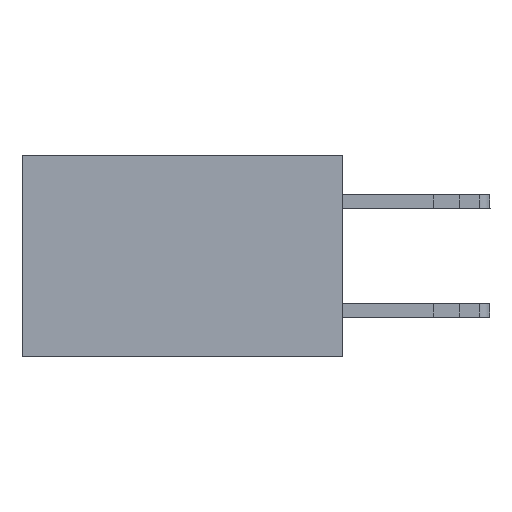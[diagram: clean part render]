
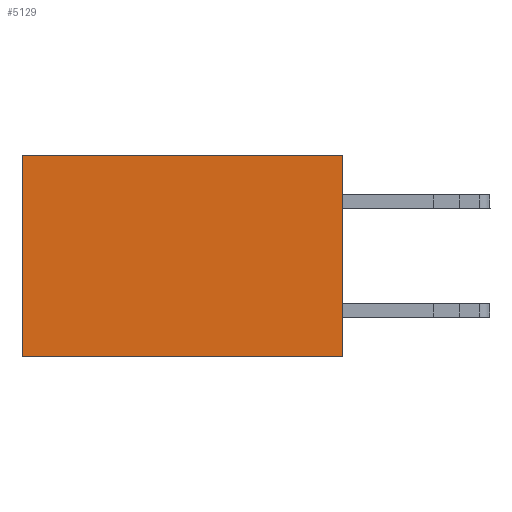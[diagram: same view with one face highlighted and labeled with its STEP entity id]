
A CAD part, left-side view. The second image highlights one B-rep face of the part: STEP entity #5129.
In plain terms, the highlighted planar face has unit normal (-1, 0, 0).
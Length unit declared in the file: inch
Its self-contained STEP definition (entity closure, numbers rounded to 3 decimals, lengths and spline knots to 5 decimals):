
#1608 = CARTESIAN_POINT ( 'NONE',  ( 0.277, 0.59, -0.37 ) ) ;
#2271 = DIRECTION ( 'NONE',  ( 0., 1., 0. ) ) ;
#2380 = DIRECTION ( 'NONE',  ( 0., 0., -1. ) ) ;
#2770 = FACE_OUTER_BOUND ( 'NONE', #17318, .T. ) ;
#4230 = AXIS2_PLACEMENT_3D ( 'NONE', #9900, #11421, #2380 ) ;
#5129 = ADVANCED_FACE ( 'NONE', ( #2770 ), #17357, .F. ) ;
#5589 = ORIENTED_EDGE ( 'NONE', *, *, #9940, .T. ) ;
#5603 = VECTOR ( 'NONE', #11030, 39.37008 ) ;
#6467 = CARTESIAN_POINT ( 'NONE',  ( 0.277, 0., -0.37 ) ) ;
#6564 = ORIENTED_EDGE ( 'NONE', *, *, #17160, .T. ) ;
#6751 = VERTEX_POINT ( 'NONE', #16392 ) ;
#8051 = DIRECTION ( 'NONE',  ( 0., 0., -1. ) ) ;
#8408 = VERTEX_POINT ( 'NONE', #9377 ) ;
#9377 = CARTESIAN_POINT ( 'NONE',  ( 0.277, 0.59, 0. ) ) ;
#9710 = LINE ( 'NONE', #18444, #5603 ) ;
#9900 = CARTESIAN_POINT ( 'NONE',  ( 0.277, 0., -0.37 ) ) ;
#9918 = CARTESIAN_POINT ( 'NONE',  ( 0.277, 0., -0.37 ) ) ;
#9940 = EDGE_CURVE ( 'NONE', #8408, #14804, #9710, .T. ) ;
#10008 = LINE ( 'NONE', #9918, #12509 ) ;
#10142 = ORIENTED_EDGE ( 'NONE', *, *, #14186, .F. ) ;
#10364 = CARTESIAN_POINT ( 'NONE',  ( 0.277, 0., -0.37 ) ) ;
#10921 = LINE ( 'NONE', #17258, #15343 ) ;
#11030 = DIRECTION ( 'NONE',  ( 0., 0., -1. ) ) ;
#11421 = DIRECTION ( 'NONE',  ( 1., 0., 0. ) ) ;
#12509 = VECTOR ( 'NONE', #12861, 39.37008 ) ;
#12861 = DIRECTION ( 'NONE',  ( 0., 1., 0. ) ) ;
#13745 = VERTEX_POINT ( 'NONE', #10364 ) ;
#14186 = EDGE_CURVE ( 'NONE', #13745, #14804, #10008, .T. ) ;
#14289 = VECTOR ( 'NONE', #8051, 39.37008 ) ;
#14804 = VERTEX_POINT ( 'NONE', #1608 ) ;
#15343 = VECTOR ( 'NONE', #2271, 39.37008 ) ;
#16354 = EDGE_CURVE ( 'NONE', #6751, #13745, #18259, .T. ) ;
#16392 = CARTESIAN_POINT ( 'NONE',  ( 0.277, 0., 0. ) ) ;
#17160 = EDGE_CURVE ( 'NONE', #6751, #8408, #10921, .T. ) ;
#17258 = CARTESIAN_POINT ( 'NONE',  ( 0.277, 0., 0. ) ) ;
#17318 = EDGE_LOOP ( 'NONE', ( #5589, #10142, #18029, #6564 ) ) ;
#17357 = PLANE ( 'NONE',  #4230 ) ;
#18029 = ORIENTED_EDGE ( 'NONE', *, *, #16354, .F. ) ;
#18259 = LINE ( 'NONE', #6467, #14289 ) ;
#18444 = CARTESIAN_POINT ( 'NONE',  ( 0.277, 0.59, -0.37 ) ) ;
